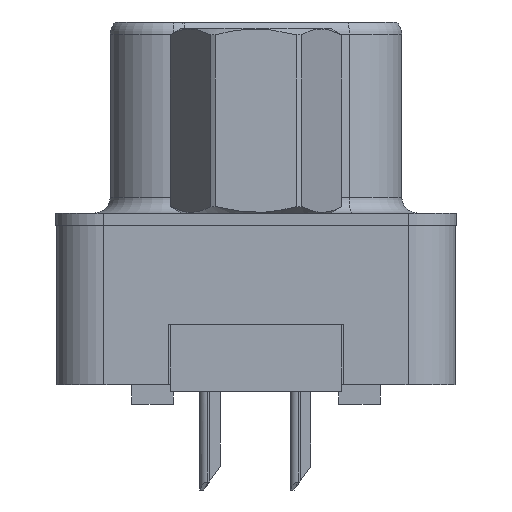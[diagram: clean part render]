
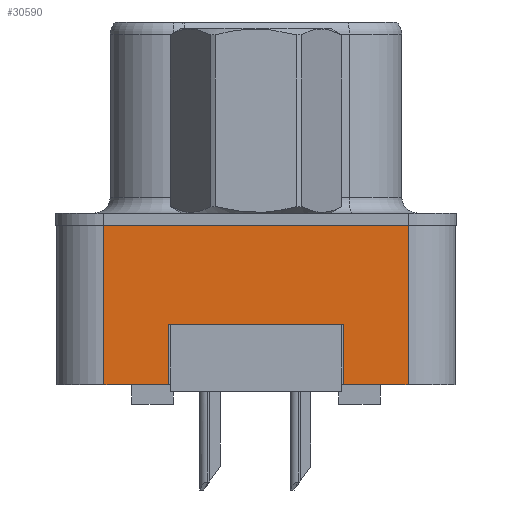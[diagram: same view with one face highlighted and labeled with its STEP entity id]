
A CAD part, left-side view. The second image highlights one B-rep face of the part: STEP entity #30590.
In plain terms, the highlighted planar face has unit normal (-1, 0, 0).
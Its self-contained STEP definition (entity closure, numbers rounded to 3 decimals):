
#21 = LINE ( 'NONE', #8139, #17214 ) ;
#205 = CARTESIAN_POINT ( 'NONE',  ( -2.91, 2.75, -3.1 ) ) ;
#728 = LINE ( 'NONE', #9194, #29078 ) ;
#784 = DIRECTION ( 'NONE',  ( 0., -1., 0. ) ) ;
#950 = CARTESIAN_POINT ( 'NONE',  ( -2.91, -4.775, -5. ) ) ;
#1008 = VERTEX_POINT ( 'NONE', #205 ) ;
#1247 = DIRECTION ( 'NONE',  ( 0., -1., 0. ) ) ;
#2372 = VECTOR ( 'NONE', #27561, 1000. ) ;
#3451 = CARTESIAN_POINT ( 'NONE',  ( -2.91, 4.775, -5. ) ) ;
#3888 = DIRECTION ( 'NONE',  ( 0., 0., 1. ) ) ;
#3894 = FACE_OUTER_BOUND ( 'NONE', #25748, .T. ) ;
#5956 = CARTESIAN_POINT ( 'NONE',  ( -2.91, 4.775, -5. ) ) ;
#6683 = CARTESIAN_POINT ( 'NONE',  ( -2.91, -4.775, 0. ) ) ;
#7196 = EDGE_CURVE ( 'NONE', #24139, #13809, #30557, .T. ) ;
#7477 = VECTOR ( 'NONE', #784, 1000. ) ;
#8139 = CARTESIAN_POINT ( 'NONE',  ( -2.91, -2.75, -3.1 ) ) ;
#8593 = EDGE_CURVE ( 'NONE', #14904, #13809, #14164, .T. ) ;
#8730 = DIRECTION ( 'NONE',  ( 0., 0., 1. ) ) ;
#8734 = CARTESIAN_POINT ( 'NONE',  ( -2.91, -4.775, -5. ) ) ;
#8833 = VERTEX_POINT ( 'NONE', #19481 ) ;
#9070 = CARTESIAN_POINT ( 'NONE',  ( -2.91, -4.775, -5. ) ) ;
#9194 = CARTESIAN_POINT ( 'NONE',  ( -2.91, 2.75, -3.1 ) ) ;
#9944 = VERTEX_POINT ( 'NONE', #5956 ) ;
#11459 = ORIENTED_EDGE ( 'NONE', *, *, #12825, .F. ) ;
#11492 = PLANE ( 'NONE',  #22562 ) ;
#11949 = DIRECTION ( 'NONE',  ( 0., 0., -1. ) ) ;
#12492 = LINE ( 'NONE', #28641, #16028 ) ;
#12825 = EDGE_CURVE ( 'NONE', #1008, #33620, #728, .T. ) ;
#13809 = VERTEX_POINT ( 'NONE', #6683 ) ;
#14023 = CARTESIAN_POINT ( 'NONE',  ( -2.91, -4.775, -5. ) ) ;
#14070 = DIRECTION ( 'NONE',  ( -1., 0., 0. ) ) ;
#14153 = LINE ( 'NONE', #3451, #2372 ) ;
#14164 = LINE ( 'NONE', #24461, #21926 ) ;
#14902 = DIRECTION ( 'NONE',  ( 0., 1., 0. ) ) ;
#14904 = VERTEX_POINT ( 'NONE', #16188 ) ;
#15676 = ORIENTED_EDGE ( 'NONE', *, *, #8593, .F. ) ;
#16028 = VECTOR ( 'NONE', #14902, 1000. ) ;
#16188 = CARTESIAN_POINT ( 'NONE',  ( -2.91, 4.775, 0. ) ) ;
#16757 = EDGE_CURVE ( 'NONE', #17767, #1008, #12492, .T. ) ;
#16823 = LINE ( 'NONE', #8734, #7477 ) ;
#17214 = VECTOR ( 'NONE', #29129, 1000. ) ;
#17767 = VERTEX_POINT ( 'NONE', #27464 ) ;
#19311 = DIRECTION ( 'NONE',  ( 0., -1., 0. ) ) ;
#19481 = CARTESIAN_POINT ( 'NONE',  ( -2.91, -2.75, -5. ) ) ;
#21635 = EDGE_CURVE ( 'NONE', #9944, #14904, #14153, .T. ) ;
#21926 = VECTOR ( 'NONE', #19311, 1000. ) ;
#22562 = AXIS2_PLACEMENT_3D ( 'NONE', #950, #14070, #8730 ) ;
#23908 = ORIENTED_EDGE ( 'NONE', *, *, #23954, .T. ) ;
#23954 = EDGE_CURVE ( 'NONE', #9944, #33620, #16823, .T. ) ;
#24139 = VERTEX_POINT ( 'NONE', #25000 ) ;
#24263 = EDGE_CURVE ( 'NONE', #8833, #24139, #26898, .T. ) ;
#24461 = CARTESIAN_POINT ( 'NONE',  ( -2.91, -4.775, 0. ) ) ;
#25000 = CARTESIAN_POINT ( 'NONE',  ( -2.91, -4.775, -5. ) ) ;
#25495 = ORIENTED_EDGE ( 'NONE', *, *, #24263, .T. ) ;
#25626 = VECTOR ( 'NONE', #1247, 1000. ) ;
#25748 = EDGE_LOOP ( 'NONE', ( #33811, #25495, #31723, #15676, #32117, #23908, #11459, #30343 ) ) ;
#26898 = LINE ( 'NONE', #14023, #25626 ) ;
#27464 = CARTESIAN_POINT ( 'NONE',  ( -2.91, -2.75, -3.1 ) ) ;
#27561 = DIRECTION ( 'NONE',  ( 0., 0., 1. ) ) ;
#28641 = CARTESIAN_POINT ( 'NONE',  ( -2.91, 2.75, -3.1 ) ) ;
#29078 = VECTOR ( 'NONE', #11949, 1000. ) ;
#29129 = DIRECTION ( 'NONE',  ( 0., 0., -1. ) ) ;
#30343 = ORIENTED_EDGE ( 'NONE', *, *, #16757, .F. ) ;
#30557 = LINE ( 'NONE', #9070, #33428 ) ;
#30590 = ADVANCED_FACE ( 'NONE', ( #3894 ), #11492, .T. ) ;
#31723 = ORIENTED_EDGE ( 'NONE', *, *, #7196, .T. ) ;
#32117 = ORIENTED_EDGE ( 'NONE', *, *, #21635, .F. ) ;
#33428 = VECTOR ( 'NONE', #3888, 1000. ) ;
#33528 = CARTESIAN_POINT ( 'NONE',  ( -2.91, 2.75, -5. ) ) ;
#33620 = VERTEX_POINT ( 'NONE', #33528 ) ;
#33811 = ORIENTED_EDGE ( 'NONE', *, *, #33946, .T. ) ;
#33946 = EDGE_CURVE ( 'NONE', #17767, #8833, #21, .T. ) ;
